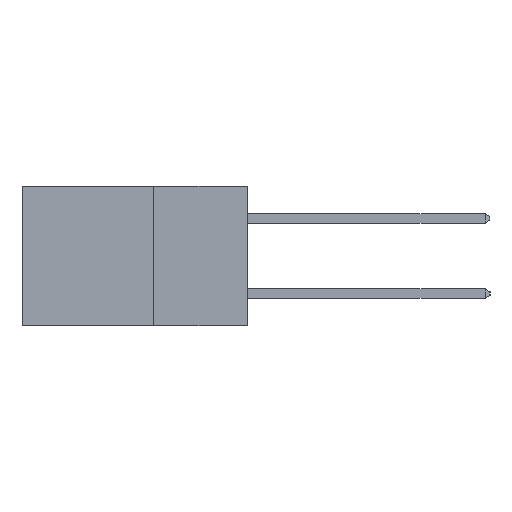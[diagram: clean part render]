
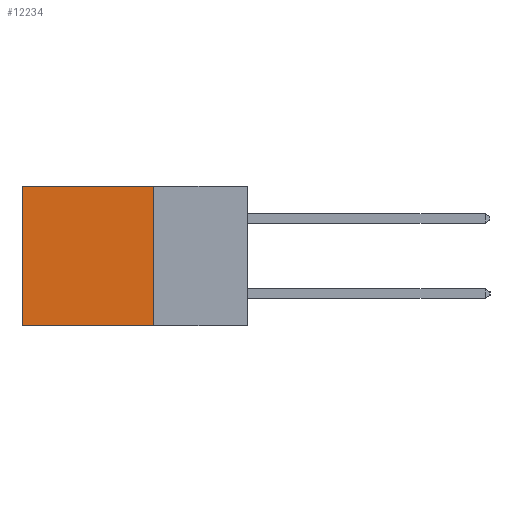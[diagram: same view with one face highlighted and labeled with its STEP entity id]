
A CAD part, left-side view. The second image highlights one B-rep face of the part: STEP entity #12234.
In plain terms, the highlighted planar face has unit normal (-1, 0, 0).
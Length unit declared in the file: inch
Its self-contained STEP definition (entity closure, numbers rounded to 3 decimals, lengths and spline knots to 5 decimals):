
#33 = CARTESIAN_POINT ( 'NONE',  ( 0.2615, 0.25, -0.37 ) ) ;
#934 = VECTOR ( 'NONE', #7622, 39.37008 ) ;
#1287 = PLANE ( 'NONE',  #7357 ) ;
#1355 = DIRECTION ( 'NONE',  ( 0., 0., -1. ) ) ;
#1502 = EDGE_CURVE ( 'NONE', #14784, #2038, #3040, .T. ) ;
#1767 = FACE_OUTER_BOUND ( 'NONE', #9885, .T. ) ;
#2038 = VERTEX_POINT ( 'NONE', #7542 ) ;
#3040 = LINE ( 'NONE', #12463, #6258 ) ;
#3335 = LINE ( 'NONE', #6351, #5793 ) ;
#3872 = VERTEX_POINT ( 'NONE', #10370 ) ;
#4264 = EDGE_CURVE ( 'NONE', #9775, #3872, #3335, .T. ) ;
#4429 = ORIENTED_EDGE ( 'NONE', *, *, #1502, .F. ) ;
#4685 = VECTOR ( 'NONE', #6983, 39.37008 ) ;
#5793 = VECTOR ( 'NONE', #7587, 39.37008 ) ;
#5997 = EDGE_CURVE ( 'NONE', #14784, #9775, #11763, .T. ) ;
#6138 = ORIENTED_EDGE ( 'NONE', *, *, #4264, .T. ) ;
#6258 = VECTOR ( 'NONE', #12270, 39.37008 ) ;
#6351 = CARTESIAN_POINT ( 'NONE',  ( 0.2615, 0.6, -0.37 ) ) ;
#6443 = CARTESIAN_POINT ( 'NONE',  ( 0.2615, 0.25, 0. ) ) ;
#6983 = DIRECTION ( 'NONE',  ( 0., 1., 0. ) ) ;
#7357 = AXIS2_PLACEMENT_3D ( 'NONE', #33, #8747, #1355 ) ;
#7542 = CARTESIAN_POINT ( 'NONE',  ( 0.2615, 0.25, -0.37 ) ) ;
#7587 = DIRECTION ( 'NONE',  ( 0., 0., -1. ) ) ;
#7622 = DIRECTION ( 'NONE',  ( 0., 1., 0. ) ) ;
#8451 = ORIENTED_EDGE ( 'NONE', *, *, #5997, .T. ) ;
#8747 = DIRECTION ( 'NONE',  ( 1., 0., 0. ) ) ;
#9552 = ORIENTED_EDGE ( 'NONE', *, *, #11643, .F. ) ;
#9775 = VERTEX_POINT ( 'NONE', #10767 ) ;
#9885 = EDGE_LOOP ( 'NONE', ( #6138, #9552, #4429, #8451 ) ) ;
#10370 = CARTESIAN_POINT ( 'NONE',  ( 0.2615, 0.6, -0.37 ) ) ;
#10767 = CARTESIAN_POINT ( 'NONE',  ( 0.2615, 0.6, 0. ) ) ;
#11643 = EDGE_CURVE ( 'NONE', #2038, #3872, #14120, .T. ) ;
#11763 = LINE ( 'NONE', #6443, #4685 ) ;
#12234 = ADVANCED_FACE ( 'NONE', ( #1767 ), #1287, .F. ) ;
#12270 = DIRECTION ( 'NONE',  ( 0., 0., -1. ) ) ;
#12463 = CARTESIAN_POINT ( 'NONE',  ( 0.2615, 0.25, -0.37 ) ) ;
#14120 = LINE ( 'NONE', #14997, #934 ) ;
#14784 = VERTEX_POINT ( 'NONE', #15301 ) ;
#14997 = CARTESIAN_POINT ( 'NONE',  ( 0.2615, 0.25, -0.37 ) ) ;
#15301 = CARTESIAN_POINT ( 'NONE',  ( 0.2615, 0.25, 0. ) ) ;
